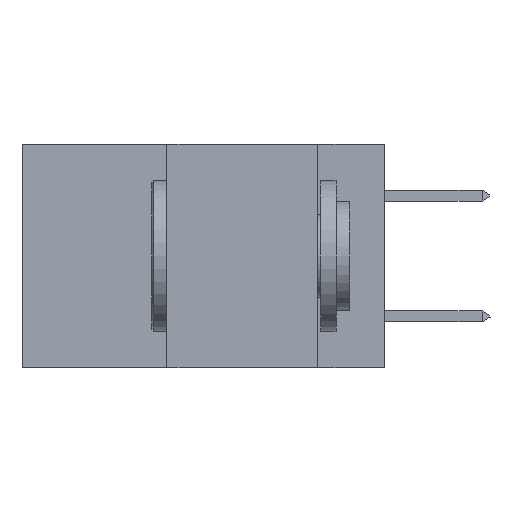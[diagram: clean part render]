
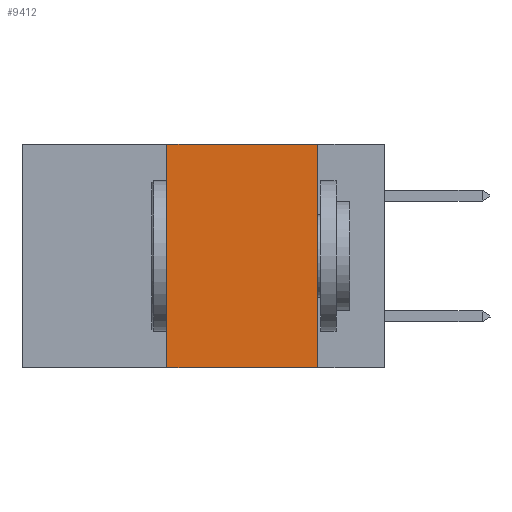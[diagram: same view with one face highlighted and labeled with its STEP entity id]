
A CAD part, left-side view. The second image highlights one B-rep face of the part: STEP entity #9412.
In plain terms, the highlighted planar face has unit normal (-1, 0, 0).
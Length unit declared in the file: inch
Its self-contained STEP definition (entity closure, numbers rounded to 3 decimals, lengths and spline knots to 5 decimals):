
#282 = AXIS2_PLACEMENT_3D ( 'NONE', #11442, #11273, #7006 ) ;
#302 = VERTEX_POINT ( 'NONE', #1225 ) ;
#760 = EDGE_CURVE ( 'NONE', #8832, #14127, #8713, .T. ) ;
#1000 = LINE ( 'NONE', #10960, #4504 ) ;
#1188 = LINE ( 'NONE', #1467, #15918 ) ;
#1225 = CARTESIAN_POINT ( 'NONE',  ( 0., 0.11, 0. ) ) ;
#1280 = DIRECTION ( 'NONE',  ( 0., -1., 0. ) ) ;
#1467 = CARTESIAN_POINT ( 'NONE',  ( 0., 0.6, 0. ) ) ;
#2192 = EDGE_CURVE ( 'NONE', #8832, #11491, #16956, .T. ) ;
#2524 = VECTOR ( 'NONE', #11756, 39.37008 ) ;
#3789 = CARTESIAN_POINT ( 'NONE',  ( 0., 0.36, -0.37 ) ) ;
#3936 = VECTOR ( 'NONE', #8418, 39.37008 ) ;
#4081 = CARTESIAN_POINT ( 'NONE',  ( 0., 0.6, -0.37 ) ) ;
#4504 = VECTOR ( 'NONE', #11024, 39.37008 ) ;
#5464 = ORIENTED_EDGE ( 'NONE', *, *, #10666, .F. ) ;
#7006 = DIRECTION ( 'NONE',  ( 0., 0., -1. ) ) ;
#7009 = CARTESIAN_POINT ( 'NONE',  ( 0., 0.11, -0.37 ) ) ;
#7070 = PLANE ( 'NONE',  #282 ) ;
#7194 = ORIENTED_EDGE ( 'NONE', *, *, #2192, .F. ) ;
#8418 = DIRECTION ( 'NONE',  ( 0., 0., 1. ) ) ;
#8713 = LINE ( 'NONE', #4081, #2524 ) ;
#8832 = VERTEX_POINT ( 'NONE', #3789 ) ;
#9386 = CARTESIAN_POINT ( 'NONE',  ( 0., 0.36, 0. ) ) ;
#9412 = ADVANCED_FACE ( 'NONE', ( #9845 ), #7070, .F. ) ;
#9845 = FACE_OUTER_BOUND ( 'NONE', #11392, .T. ) ;
#10666 = EDGE_CURVE ( 'NONE', #302, #14127, #1000, .T. ) ;
#10960 = CARTESIAN_POINT ( 'NONE',  ( 0., 0.11, 0. ) ) ;
#11024 = DIRECTION ( 'NONE',  ( 0., 0., -1. ) ) ;
#11273 = DIRECTION ( 'NONE',  ( 1., 0., 0. ) ) ;
#11328 = EDGE_CURVE ( 'NONE', #11491, #302, #1188, .T. ) ;
#11392 = EDGE_LOOP ( 'NONE', ( #5464, #13613, #7194, #11704 ) ) ;
#11442 = CARTESIAN_POINT ( 'NONE',  ( 0., 0.6, 0. ) ) ;
#11491 = VERTEX_POINT ( 'NONE', #15752 ) ;
#11704 = ORIENTED_EDGE ( 'NONE', *, *, #760, .T. ) ;
#11756 = DIRECTION ( 'NONE',  ( 0., -1., 0. ) ) ;
#13613 = ORIENTED_EDGE ( 'NONE', *, *, #11328, .F. ) ;
#14127 = VERTEX_POINT ( 'NONE', #7009 ) ;
#15752 = CARTESIAN_POINT ( 'NONE',  ( 0., 0.36, 0. ) ) ;
#15918 = VECTOR ( 'NONE', #1280, 39.37008 ) ;
#16956 = LINE ( 'NONE', #9386, #3936 ) ;
